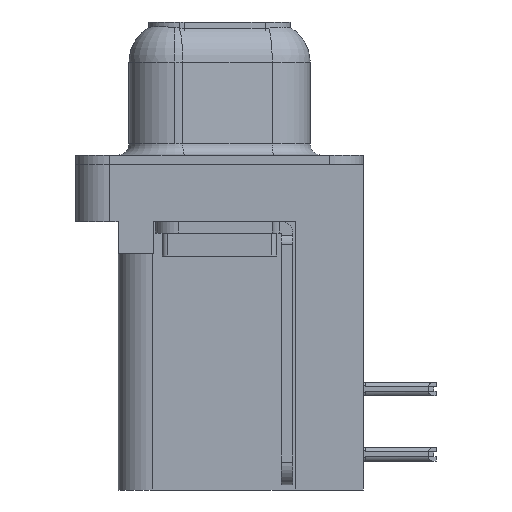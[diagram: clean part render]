
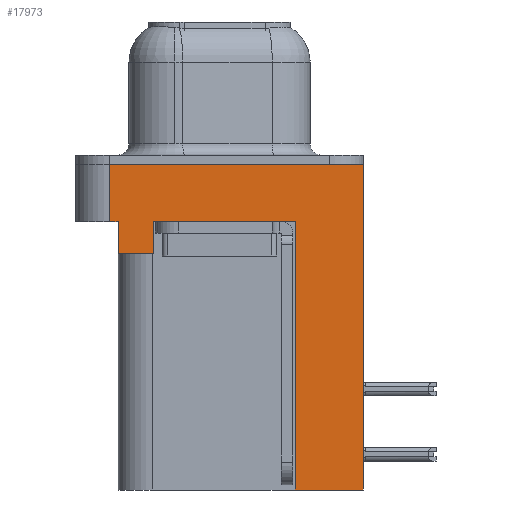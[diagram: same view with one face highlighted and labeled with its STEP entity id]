
A CAD part, left-side view. The second image highlights one B-rep face of the part: STEP entity #17973.
In plain terms, the highlighted planar face has unit normal (-1, 0, 0).
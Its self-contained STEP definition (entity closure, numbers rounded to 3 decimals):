
#1311 = CARTESIAN_POINT ( 'NONE',  ( -2.935, 4.775, -2.5 ) ) ;
#1627 = LINE ( 'NONE', #15852, #18389 ) ;
#1638 = ORIENTED_EDGE ( 'NONE', *, *, #25194, .F. ) ;
#1744 = EDGE_CURVE ( 'NONE', #23778, #23513, #8158, .T. ) ;
#1962 = VERTEX_POINT ( 'NONE', #5075 ) ;
#2064 = CARTESIAN_POINT ( 'NONE',  ( -2.935, 2.895, -2.5 ) ) ;
#2133 = EDGE_CURVE ( 'NONE', #6355, #20471, #21370, .T. ) ;
#2518 = LINE ( 'NONE', #9220, #9229 ) ;
#2991 = DIRECTION ( 'NONE',  ( 0., 0., 1. ) ) ;
#3674 = CARTESIAN_POINT ( 'NONE',  ( -2.935, -3.295, -14.2 ) ) ;
#3741 = EDGE_CURVE ( 'NONE', #20471, #6868, #3891, .T. ) ;
#3752 = ORIENTED_EDGE ( 'NONE', *, *, #19995, .T. ) ;
#3891 = LINE ( 'NONE', #5775, #16391 ) ;
#4556 = CARTESIAN_POINT ( 'NONE',  ( -2.935, 4.425, -3.9 ) ) ;
#5059 = PLANE ( 'NONE',  #11830 ) ;
#5075 = CARTESIAN_POINT ( 'NONE',  ( -2.935, 4.425, -3.9 ) ) ;
#5775 = CARTESIAN_POINT ( 'NONE',  ( -2.935, -6.275, -2.5 ) ) ;
#5829 = ORIENTED_EDGE ( 'NONE', *, *, #15658, .F. ) ;
#6355 = VERTEX_POINT ( 'NONE', #15011 ) ;
#6665 = FACE_OUTER_BOUND ( 'NONE', #25922, .T. ) ;
#6868 = VERTEX_POINT ( 'NONE', #25461 ) ;
#7017 = CARTESIAN_POINT ( 'NONE',  ( -2.935, 2.895, -3.9 ) ) ;
#7652 = LINE ( 'NONE', #13813, #21771 ) ;
#8000 = VECTOR ( 'NONE', #18375, 1000. ) ;
#8158 = LINE ( 'NONE', #8286, #12693 ) ;
#8286 = CARTESIAN_POINT ( 'NONE',  ( -2.935, -6.275, 0. ) ) ;
#9220 = CARTESIAN_POINT ( 'NONE',  ( -2.935, -6.275, -2.5 ) ) ;
#9229 = VECTOR ( 'NONE', #10679, 1000. ) ;
#9649 = ORIENTED_EDGE ( 'NONE', *, *, #17163, .F. ) ;
#10679 = DIRECTION ( 'NONE',  ( 0., 0., 1. ) ) ;
#11212 = CARTESIAN_POINT ( 'NONE',  ( -2.935, -6.275, -2.5 ) ) ;
#11310 = ORIENTED_EDGE ( 'NONE', *, *, #17510, .F. ) ;
#11522 = DIRECTION ( 'NONE',  ( 0., 1., 0. ) ) ;
#11585 = VERTEX_POINT ( 'NONE', #1311 ) ;
#11650 = LINE ( 'NONE', #19844, #25050 ) ;
#11830 = AXIS2_PLACEMENT_3D ( 'NONE', #11212, #20889, #17123 ) ;
#12191 = DIRECTION ( 'NONE',  ( 0., 0., 1. ) ) ;
#12250 = VECTOR ( 'NONE', #11522, 1000. ) ;
#12693 = VECTOR ( 'NONE', #18484, 1000. ) ;
#13281 = VECTOR ( 'NONE', #2991, 1000. ) ;
#13494 = DIRECTION ( 'NONE',  ( 0., -1., 0. ) ) ;
#13668 = LINE ( 'NONE', #21870, #12250 ) ;
#13813 = CARTESIAN_POINT ( 'NONE',  ( -2.935, 4.775, -2.5 ) ) ;
#13974 = ORIENTED_EDGE ( 'NONE', *, *, #14174, .T. ) ;
#14174 = EDGE_CURVE ( 'NONE', #20814, #23513, #2518, .T. ) ;
#14366 = CARTESIAN_POINT ( 'NONE',  ( -2.935, -6.275, -14.2 ) ) ;
#14817 = VERTEX_POINT ( 'NONE', #3674 ) ;
#15011 = CARTESIAN_POINT ( 'NONE',  ( -2.935, 2.895, -3.9 ) ) ;
#15519 = CARTESIAN_POINT ( 'NONE',  ( -2.935, -6.275, -2.5 ) ) ;
#15658 = EDGE_CURVE ( 'NONE', #14817, #6868, #11650, .T. ) ;
#15852 = CARTESIAN_POINT ( 'NONE',  ( -2.935, 4.425, -3.9 ) ) ;
#15902 = VERTEX_POINT ( 'NONE', #24068 ) ;
#16391 = VECTOR ( 'NONE', #22142, 1000. ) ;
#17123 = DIRECTION ( 'NONE',  ( 0., 0., 1. ) ) ;
#17163 = EDGE_CURVE ( 'NONE', #20814, #14817, #13668, .T. ) ;
#17510 = EDGE_CURVE ( 'NONE', #1962, #15902, #22797, .T. ) ;
#17862 = DIRECTION ( 'NONE',  ( 0., 1., 0. ) ) ;
#17973 = ADVANCED_FACE ( 'NONE', ( #6665 ), #5059, .T. ) ;
#18375 = DIRECTION ( 'NONE',  ( 0., 0., 1. ) ) ;
#18389 = VECTOR ( 'NONE', #17862, 1000. ) ;
#18484 = DIRECTION ( 'NONE',  ( 0., -1., 0. ) ) ;
#18717 = VECTOR ( 'NONE', #13494, 1000. ) ;
#19759 = ORIENTED_EDGE ( 'NONE', *, *, #2133, .T. ) ;
#19844 = CARTESIAN_POINT ( 'NONE',  ( -2.935, -3.295, -14.2 ) ) ;
#19995 = EDGE_CURVE ( 'NONE', #11585, #15902, #26117, .T. ) ;
#20428 = CARTESIAN_POINT ( 'NONE',  ( -2.935, 4.775, 0. ) ) ;
#20471 = VERTEX_POINT ( 'NONE', #2064 ) ;
#20814 = VERTEX_POINT ( 'NONE', #14366 ) ;
#20889 = DIRECTION ( 'NONE',  ( -1., 0., 0. ) ) ;
#20988 = CARTESIAN_POINT ( 'NONE',  ( -2.935, -6.275, 0. ) ) ;
#21241 = EDGE_CURVE ( 'NONE', #11585, #23778, #7652, .T. ) ;
#21370 = LINE ( 'NONE', #7017, #13281 ) ;
#21771 = VECTOR ( 'NONE', #12191, 1000. ) ;
#21870 = CARTESIAN_POINT ( 'NONE',  ( -2.935, -3.295, -14.2 ) ) ;
#22142 = DIRECTION ( 'NONE',  ( 0., -1., 0. ) ) ;
#22778 = DIRECTION ( 'NONE',  ( 0., 0., 1. ) ) ;
#22797 = LINE ( 'NONE', #4556, #8000 ) ;
#23513 = VERTEX_POINT ( 'NONE', #20988 ) ;
#23614 = ORIENTED_EDGE ( 'NONE', *, *, #21241, .F. ) ;
#23778 = VERTEX_POINT ( 'NONE', #20428 ) ;
#24068 = CARTESIAN_POINT ( 'NONE',  ( -2.935, 4.425, -2.5 ) ) ;
#25050 = VECTOR ( 'NONE', #22778, 1000. ) ;
#25194 = EDGE_CURVE ( 'NONE', #6355, #1962, #1627, .T. ) ;
#25461 = CARTESIAN_POINT ( 'NONE',  ( -2.935, -3.295, -2.5 ) ) ;
#25580 = ORIENTED_EDGE ( 'NONE', *, *, #3741, .T. ) ;
#25922 = EDGE_LOOP ( 'NONE', ( #26250, #23614, #3752, #11310, #1638, #19759, #25580, #5829, #9649, #13974 ) ) ;
#26117 = LINE ( 'NONE', #15519, #18717 ) ;
#26250 = ORIENTED_EDGE ( 'NONE', *, *, #1744, .F. ) ;
